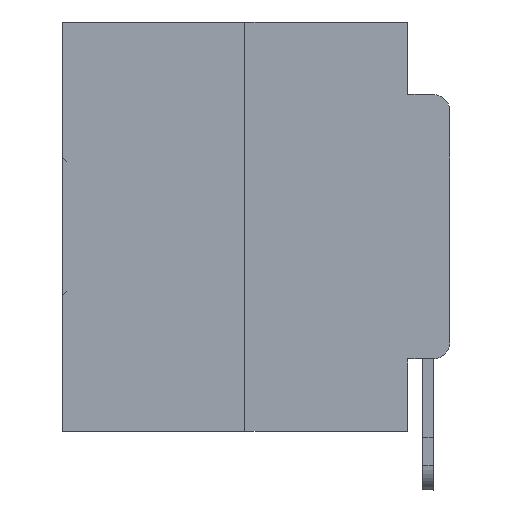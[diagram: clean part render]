
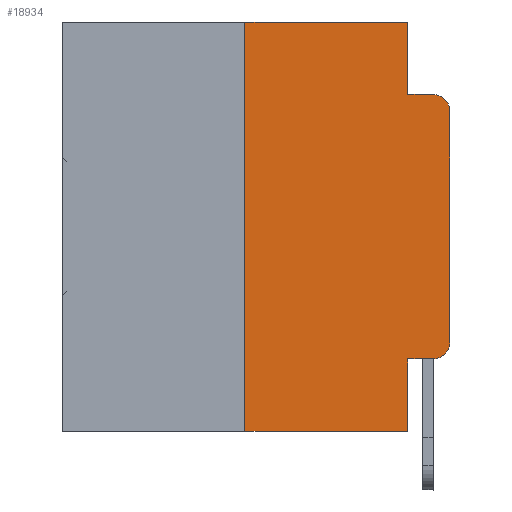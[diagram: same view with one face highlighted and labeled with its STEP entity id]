
A CAD part, left-side view. The second image highlights one B-rep face of the part: STEP entity #18934.
In plain terms, the highlighted planar face has unit normal (-1, 0, 0).
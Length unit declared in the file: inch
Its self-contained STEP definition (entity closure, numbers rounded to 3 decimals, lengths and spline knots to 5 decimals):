
#957 = DIRECTION ( 'NONE',  ( 0., 0., -1. ) ) ;
#1108 = DIRECTION ( 'NONE',  ( 0., 0., -1. ) ) ;
#1161 = VERTEX_POINT ( 'NONE', #19980 ) ;
#1337 = DIRECTION ( 'NONE',  ( 0., 0., 1. ) ) ;
#1838 = LINE ( 'NONE', #21774, #9068 ) ;
#2286 = LINE ( 'NONE', #26952, #32156 ) ;
#2430 = DIRECTION ( 'NONE',  ( -1., 0., 0. ) ) ;
#2668 = EDGE_CURVE ( 'NONE', #1161, #4134, #1838, .T. ) ;
#3374 = CARTESIAN_POINT ( 'NONE',  ( 0., 0., -0.1085 ) ) ;
#3615 = ORIENTED_EDGE ( 'NONE', *, *, #22431, .F. ) ;
#3808 = CARTESIAN_POINT ( 'NONE',  ( 0., 0.051, 0. ) ) ;
#4134 = VERTEX_POINT ( 'NONE', #4177 ) ;
#4177 = CARTESIAN_POINT ( 'NONE',  ( 0., 0.051, -0.5 ) ) ;
#4354 = LINE ( 'NONE', #31310, #14116 ) ;
#4606 = DIRECTION ( 'NONE',  ( 0., 0., -1. ) ) ;
#4725 = ORIENTED_EDGE ( 'NONE', *, *, #2668, .T. ) ;
#5209 = CARTESIAN_POINT ( 'NONE',  ( 0., 0.02, -0.1085 ) ) ;
#5378 = VERTEX_POINT ( 'NONE', #21456 ) ;
#5606 = VERTEX_POINT ( 'NONE', #29460 ) ;
#5881 = EDGE_LOOP ( 'NONE', ( #10088, #6089, #9337, #18354, #3615, #30879, #4725, #19781, #14195, #17691 ) ) ;
#6089 = ORIENTED_EDGE ( 'NONE', *, *, #13498, .T. ) ;
#6122 = DIRECTION ( 'NONE',  ( 0., -1., 0. ) ) ;
#7022 = AXIS2_PLACEMENT_3D ( 'NONE', #5209, #2430, #15495 ) ;
#9068 = VECTOR ( 'NONE', #6122, 39.37008 ) ;
#9337 = ORIENTED_EDGE ( 'NONE', *, *, #31202, .F. ) ;
#10088 = ORIENTED_EDGE ( 'NONE', *, *, #25241, .T. ) ;
#10676 = EDGE_CURVE ( 'NONE', #1161, #19398, #32700, .T. ) ;
#10910 = EDGE_CURVE ( 'NONE', #13482, #11524, #13214, .T. ) ;
#11180 = CARTESIAN_POINT ( 'NONE',  ( 0., 0.25, 0. ) ) ;
#11524 = VERTEX_POINT ( 'NONE', #14177 ) ;
#11595 = CARTESIAN_POINT ( 'NONE',  ( 0., 0.051, -0.0885 ) ) ;
#11759 = EDGE_CURVE ( 'NONE', #5606, #17453, #22681, .T. ) ;
#11869 = DIRECTION ( 'NONE',  ( -1., 0., 0. ) ) ;
#12165 = VECTOR ( 'NONE', #1108, 39.37008 ) ;
#12206 = CIRCLE ( 'NONE', #22115, 0.02 ) ;
#12598 = VERTEX_POINT ( 'NONE', #3374 ) ;
#13214 = LINE ( 'NONE', #20697, #29484 ) ;
#13482 = VERTEX_POINT ( 'NONE', #28204 ) ;
#13498 = EDGE_CURVE ( 'NONE', #12598, #20913, #25334, .T. ) ;
#14116 = VECTOR ( 'NONE', #25892, 39.37008 ) ;
#14177 = CARTESIAN_POINT ( 'NONE',  ( 0., 0.02, -0.4115 ) ) ;
#14195 = ORIENTED_EDGE ( 'NONE', *, *, #10910, .T. ) ;
#14400 = LINE ( 'NONE', #19241, #22319 ) ;
#15495 = DIRECTION ( 'NONE',  ( 0., 0., -1. ) ) ;
#15659 = EDGE_CURVE ( 'NONE', #13482, #4134, #28377, .T. ) ;
#16661 = CARTESIAN_POINT ( 'NONE',  ( 0., 0.473, 0. ) ) ;
#16890 = VECTOR ( 'NONE', #31843, 39.37008 ) ;
#17453 = VERTEX_POINT ( 'NONE', #11595 ) ;
#17691 = ORIENTED_EDGE ( 'NONE', *, *, #27107, .T. ) ;
#18319 = FACE_OUTER_BOUND ( 'NONE', #5881, .T. ) ;
#18354 = ORIENTED_EDGE ( 'NONE', *, *, #11759, .F. ) ;
#18934 = ADVANCED_FACE ( 'NONE', ( #18319 ), #31447, .F. ) ;
#18991 = DIRECTION ( 'NONE',  ( 1., 0., 0. ) ) ;
#19241 = CARTESIAN_POINT ( 'NONE',  ( 0., 0., 0. ) ) ;
#19398 = VERTEX_POINT ( 'NONE', #11180 ) ;
#19781 = ORIENTED_EDGE ( 'NONE', *, *, #15659, .F. ) ;
#19980 = CARTESIAN_POINT ( 'NONE',  ( 0., 0.25, -0.5 ) ) ;
#20697 = CARTESIAN_POINT ( 'NONE',  ( 0., 0.051, -0.4115 ) ) ;
#20913 = VERTEX_POINT ( 'NONE', #27962 ) ;
#21456 = CARTESIAN_POINT ( 'NONE',  ( 0., 0., -0.3915 ) ) ;
#21774 = CARTESIAN_POINT ( 'NONE',  ( 0., 0.473, -0.5 ) ) ;
#22115 = AXIS2_PLACEMENT_3D ( 'NONE', #32405, #11869, #4606 ) ;
#22319 = VECTOR ( 'NONE', #1337, 39.37008 ) ;
#22431 = EDGE_CURVE ( 'NONE', #19398, #5606, #4354, .T. ) ;
#22681 = LINE ( 'NONE', #30192, #31365 ) ;
#24107 = CARTESIAN_POINT ( 'NONE',  ( 0., 0.25, 0. ) ) ;
#25241 = EDGE_CURVE ( 'NONE', #5378, #12598, #14400, .T. ) ;
#25334 = CIRCLE ( 'NONE', #7022, 0.02 ) ;
#25892 = DIRECTION ( 'NONE',  ( 0., -1., 0. ) ) ;
#26952 = CARTESIAN_POINT ( 'NONE',  ( 0., 0.051, -0.0885 ) ) ;
#27107 = EDGE_CURVE ( 'NONE', #11524, #5378, #12206, .T. ) ;
#27634 = DIRECTION ( 'NONE',  ( 0., 0., -1. ) ) ;
#27962 = CARTESIAN_POINT ( 'NONE',  ( 0., 0.02, -0.0885 ) ) ;
#27988 = DIRECTION ( 'NONE',  ( 0., -1., 0. ) ) ;
#28204 = CARTESIAN_POINT ( 'NONE',  ( 0., 0.051, -0.4115 ) ) ;
#28377 = LINE ( 'NONE', #3808, #12165 ) ;
#29460 = CARTESIAN_POINT ( 'NONE',  ( 0., 0.051, 0. ) ) ;
#29484 = VECTOR ( 'NONE', #27988, 39.37008 ) ;
#30192 = CARTESIAN_POINT ( 'NONE',  ( 0., 0.051, 0. ) ) ;
#30879 = ORIENTED_EDGE ( 'NONE', *, *, #10676, .F. ) ;
#31202 = EDGE_CURVE ( 'NONE', #17453, #20913, #2286, .T. ) ;
#31310 = CARTESIAN_POINT ( 'NONE',  ( 0., 0.473, 0. ) ) ;
#31365 = VECTOR ( 'NONE', #27634, 39.37008 ) ;
#31447 = PLANE ( 'NONE',  #31861 ) ;
#31843 = DIRECTION ( 'NONE',  ( 0., 0., 1. ) ) ;
#31861 = AXIS2_PLACEMENT_3D ( 'NONE', #16661, #18991, #957 ) ;
#31964 = DIRECTION ( 'NONE',  ( 0., -1., 0. ) ) ;
#32156 = VECTOR ( 'NONE', #31964, 39.37008 ) ;
#32405 = CARTESIAN_POINT ( 'NONE',  ( 0., 0.02, -0.3915 ) ) ;
#32700 = LINE ( 'NONE', #24107, #16890 ) ;
